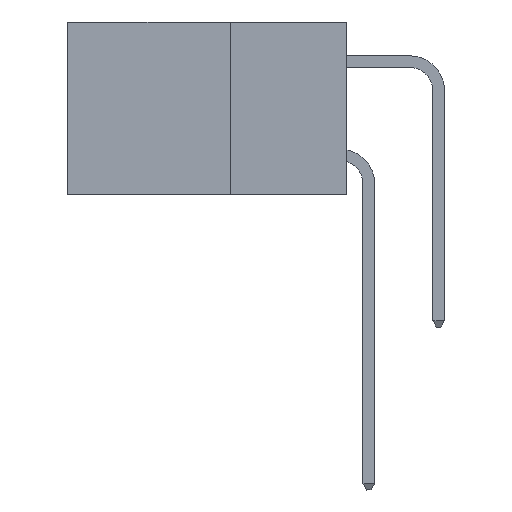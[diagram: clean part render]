
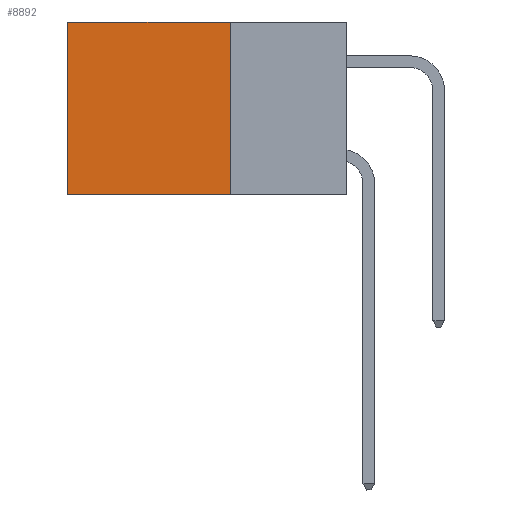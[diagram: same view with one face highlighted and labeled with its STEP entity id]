
A CAD part, left-side view. The second image highlights one B-rep face of the part: STEP entity #8892.
In plain terms, the highlighted planar face has unit normal (-1, 0, 0).
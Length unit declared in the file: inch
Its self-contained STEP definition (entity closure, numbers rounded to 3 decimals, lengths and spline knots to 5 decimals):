
#987 = CARTESIAN_POINT ( 'NONE',  ( 0.2875, 0.6, 0. ) ) ;
#2001 = VECTOR ( 'NONE', #11451, 39.37008 ) ;
#2375 = DIRECTION ( 'NONE',  ( 1., 0., 0. ) ) ;
#2535 = CARTESIAN_POINT ( 'NONE',  ( 0.2875, 0.25, 0. ) ) ;
#2778 = CARTESIAN_POINT ( 'NONE',  ( 0.2875, 0.25, 0. ) ) ;
#2807 = DIRECTION ( 'NONE',  ( 0., 0., -1. ) ) ;
#3056 = FACE_OUTER_BOUND ( 'NONE', #14007, .T. ) ;
#3332 = CARTESIAN_POINT ( 'NONE',  ( 0.2875, 0.25, 0. ) ) ;
#3855 = ORIENTED_EDGE ( 'NONE', *, *, #15761, .T. ) ;
#4012 = CARTESIAN_POINT ( 'NONE',  ( 0.2875, 0.25, -0.37 ) ) ;
#4705 = VECTOR ( 'NONE', #11082, 39.37008 ) ;
#7919 = VERTEX_POINT ( 'NONE', #12509 ) ;
#8892 = ADVANCED_FACE ( 'NONE', ( #3056 ), #11499, .F. ) ;
#8948 = LINE ( 'NONE', #10091, #2001 ) ;
#10011 = LINE ( 'NONE', #11871, #13977 ) ;
#10091 = CARTESIAN_POINT ( 'NONE',  ( 0.2875, 0.6, 0. ) ) ;
#10592 = LINE ( 'NONE', #11838, #15740 ) ;
#11082 = DIRECTION ( 'NONE',  ( 0., 1., 0. ) ) ;
#11451 = DIRECTION ( 'NONE',  ( 0., 0., -1. ) ) ;
#11499 = PLANE ( 'NONE',  #12769 ) ;
#11774 = DIRECTION ( 'NONE',  ( 0., 1., 0. ) ) ;
#11838 = CARTESIAN_POINT ( 'NONE',  ( 0.2875, 0.25, -0.37 ) ) ;
#11871 = CARTESIAN_POINT ( 'NONE',  ( 0.2875, 0.25, 0. ) ) ;
#12326 = LINE ( 'NONE', #3332, #4705 ) ;
#12509 = CARTESIAN_POINT ( 'NONE',  ( 0.2875, 0.6, -0.37 ) ) ;
#12769 = AXIS2_PLACEMENT_3D ( 'NONE', #2778, #2375, #14523 ) ;
#13977 = VECTOR ( 'NONE', #2807, 39.37008 ) ;
#14007 = EDGE_LOOP ( 'NONE', ( #14958, #16030, #16182, #3855 ) ) ;
#14194 = VERTEX_POINT ( 'NONE', #987 ) ;
#14523 = DIRECTION ( 'NONE',  ( 0., 0., -1. ) ) ;
#14816 = VERTEX_POINT ( 'NONE', #4012 ) ;
#14958 = ORIENTED_EDGE ( 'NONE', *, *, #18559, .T. ) ;
#15441 = EDGE_CURVE ( 'NONE', #16145, #14816, #10011, .T. ) ;
#15740 = VECTOR ( 'NONE', #11774, 39.37008 ) ;
#15761 = EDGE_CURVE ( 'NONE', #16145, #14194, #12326, .T. ) ;
#16030 = ORIENTED_EDGE ( 'NONE', *, *, #18665, .F. ) ;
#16145 = VERTEX_POINT ( 'NONE', #2535 ) ;
#16182 = ORIENTED_EDGE ( 'NONE', *, *, #15441, .F. ) ;
#18559 = EDGE_CURVE ( 'NONE', #14194, #7919, #8948, .T. ) ;
#18665 = EDGE_CURVE ( 'NONE', #14816, #7919, #10592, .T. ) ;
